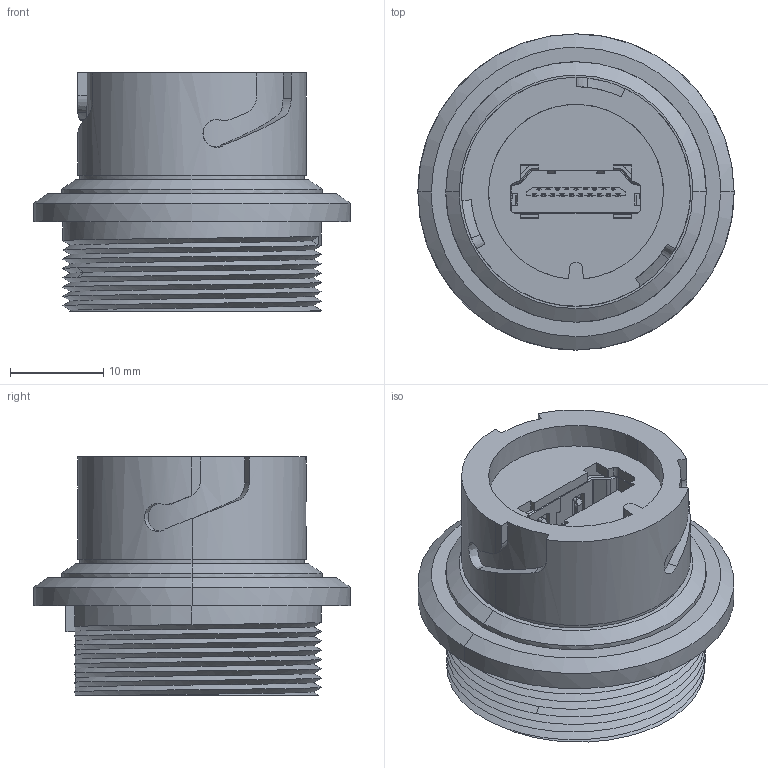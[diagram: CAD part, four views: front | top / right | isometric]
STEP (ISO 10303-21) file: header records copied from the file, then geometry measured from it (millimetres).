
FILE_DESCRIPTION (( 'STEP AP214' ), '1' );
FILE_NAME ('694-W19-660-012.STEP', '2021-06-09T15:13:16', ( '' ), ( '' ), 'SwSTEP 2.0', 'SolidWorks 2020', '' );
FILE_SCHEMA (( 'AUTOMOTIVE_DESIGN' ));
Length unit declared in the file: millimetre
Products named in the file (8): HDMI ASSY 694-W19-X60-012; HOUSING 694-W19-X60-012; 694-W19-660-012; HDMI HOUSING1 694-W19-X60-012; HDMI HOUSING2 694-W19-X60-012; HDMI CONTACT2 694-W19-X60-012; HDMI CONTACT1 694-W19-X60-012; HDMI SHELL 694-W19-X60-012
Assembly tree (24 placements, depth 3):
  694-W19-660-012
    HDMI ASSY 694-W19-X60-012
      HDMI HOUSING1 694-W19-X60-012
      HDMI HOUSING2 694-W19-X60-012
      HDMI CONTACT1 694-W19-X60-012  x9
      HDMI CONTACT2 694-W19-X60-012  x10
      HDMI SHELL 694-W19-X60-012
    HOUSING 694-W19-X60-012
Bounding box: 34 x 34 x 25.6 mm (x, y, z)
Volume: 7371.3 mm3; surface area: 9732.3 mm2
Topology: 23 solids, 23 shells, 1962 faces, 5736 edges, 3786 vertices
Faces by surface type: plane 1365, cylinder 542, bspline 43, cone 12
Entity records: 46915 total; most frequent: CARTESIAN_POINT 18404, ORIENTED_EDGE 6372, DIRECTION 5062, EDGE_CURVE 3186, LINE 2600, VECTOR 2600, VERTEX_POINT 2086, AXIS2_PLACEMENT_3D 1231
